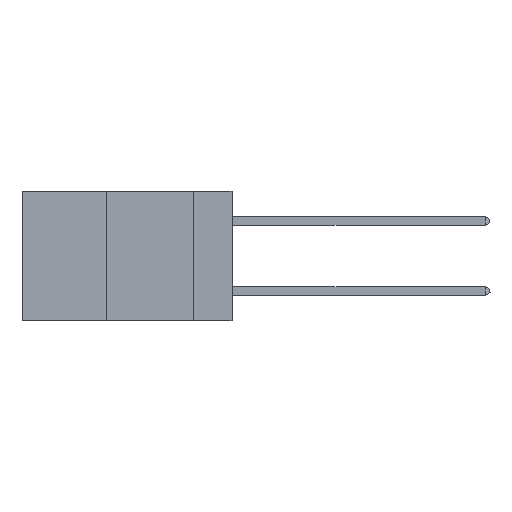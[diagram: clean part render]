
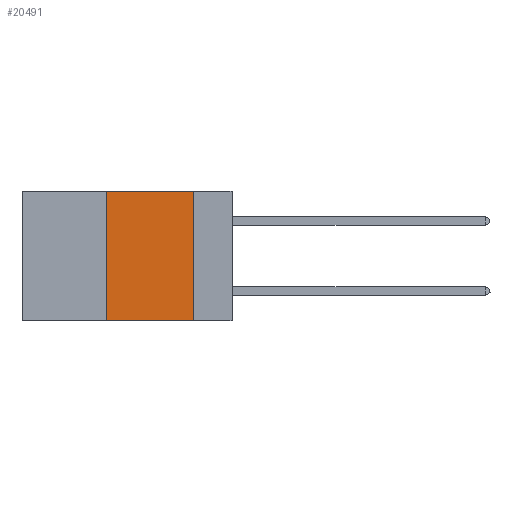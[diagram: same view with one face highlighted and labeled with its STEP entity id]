
A CAD part, left-side view. The second image highlights one B-rep face of the part: STEP entity #20491.
In plain terms, the highlighted planar face has unit normal (-1, 0, 0).
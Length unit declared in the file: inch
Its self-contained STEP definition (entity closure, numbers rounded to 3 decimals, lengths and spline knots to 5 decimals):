
#812 = EDGE_LOOP ( 'NONE', ( #29843, #24229, #6457, #7045 ) ) ;
#1657 = AXIS2_PLACEMENT_3D ( 'NONE', #4520, #17352, #34231 ) ;
#1687 = LINE ( 'NONE', #24930, #6833 ) ;
#1993 = DIRECTION ( 'NONE',  ( 0., 0., 1. ) ) ;
#4104 = LINE ( 'NONE', #8080, #17490 ) ;
#4520 = CARTESIAN_POINT ( 'NONE',  ( 0., 0.6, 0. ) ) ;
#5345 = DIRECTION ( 'NONE',  ( 0., 0., -1. ) ) ;
#5415 = EDGE_CURVE ( 'NONE', #6977, #15181, #1687, .T. ) ;
#5454 = DIRECTION ( 'NONE',  ( 0., -1., 0. ) ) ;
#6447 = CARTESIAN_POINT ( 'NONE',  ( 0., 0.36, -0.37 ) ) ;
#6457 = ORIENTED_EDGE ( 'NONE', *, *, #18591, .F. ) ;
#6833 = VECTOR ( 'NONE', #5345, 39.37008 ) ;
#6977 = VERTEX_POINT ( 'NONE', #18892 ) ;
#7045 = ORIENTED_EDGE ( 'NONE', *, *, #32379, .T. ) ;
#8080 = CARTESIAN_POINT ( 'NONE',  ( 0., 0.6, -0.37 ) ) ;
#8915 = CARTESIAN_POINT ( 'NONE',  ( 0., 0.6, 0. ) ) ;
#11538 = DIRECTION ( 'NONE',  ( 0., -1., 0. ) ) ;
#12195 = VECTOR ( 'NONE', #1993, 39.37008 ) ;
#13202 = CARTESIAN_POINT ( 'NONE',  ( 0., 0.36, 0. ) ) ;
#15181 = VERTEX_POINT ( 'NONE', #25378 ) ;
#17352 = DIRECTION ( 'NONE',  ( 1., 0., 0. ) ) ;
#17490 = VECTOR ( 'NONE', #11538, 39.37008 ) ;
#18591 = EDGE_CURVE ( 'NONE', #33298, #33496, #40629, .T. ) ;
#18892 = CARTESIAN_POINT ( 'NONE',  ( 0., 0.11, 0. ) ) ;
#20491 = ADVANCED_FACE ( 'NONE', ( #22468 ), #30919, .F. ) ;
#20624 = EDGE_CURVE ( 'NONE', #33496, #6977, #38511, .T. ) ;
#22468 = FACE_OUTER_BOUND ( 'NONE', #812, .T. ) ;
#24229 = ORIENTED_EDGE ( 'NONE', *, *, #20624, .F. ) ;
#24930 = CARTESIAN_POINT ( 'NONE',  ( 0., 0.11, 0. ) ) ;
#25378 = CARTESIAN_POINT ( 'NONE',  ( 0., 0.11, -0.37 ) ) ;
#29843 = ORIENTED_EDGE ( 'NONE', *, *, #5415, .F. ) ;
#30919 = PLANE ( 'NONE',  #1657 ) ;
#32379 = EDGE_CURVE ( 'NONE', #33298, #15181, #4104, .T. ) ;
#33298 = VERTEX_POINT ( 'NONE', #6447 ) ;
#33496 = VERTEX_POINT ( 'NONE', #13202 ) ;
#34231 = DIRECTION ( 'NONE',  ( 0., 0., -1. ) ) ;
#38511 = LINE ( 'NONE', #8915, #42588 ) ;
#40629 = LINE ( 'NONE', #41343, #12195 ) ;
#41343 = CARTESIAN_POINT ( 'NONE',  ( 0., 0.36, 0. ) ) ;
#42588 = VECTOR ( 'NONE', #5454, 39.37008 ) ;
